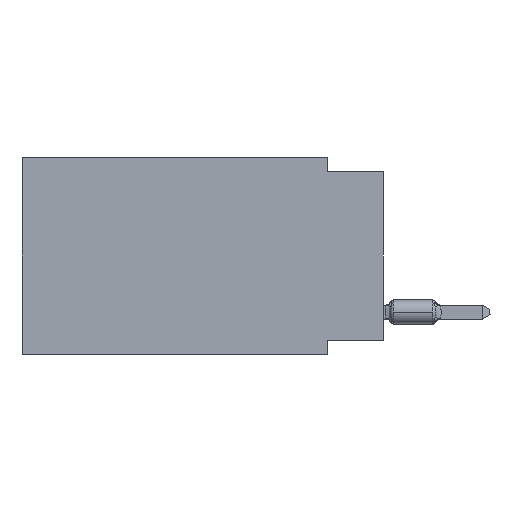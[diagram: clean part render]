
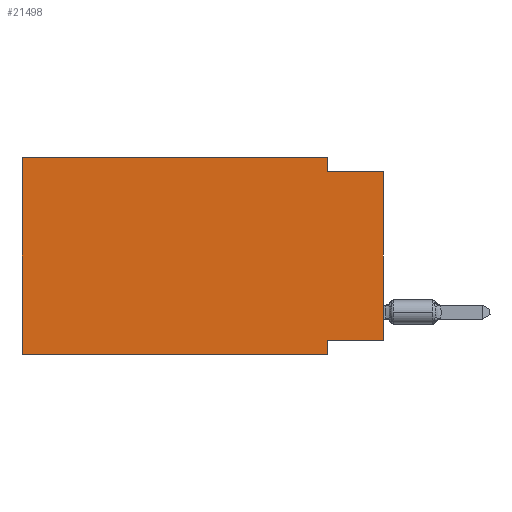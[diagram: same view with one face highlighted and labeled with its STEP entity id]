
A CAD part, left-side view. The second image highlights one B-rep face of the part: STEP entity #21498.
In plain terms, the highlighted planar face has unit normal (-1, 0, 0).
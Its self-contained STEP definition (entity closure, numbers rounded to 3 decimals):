
#720 = CARTESIAN_POINT ( 'NONE',  ( 0., 2.54, -8.255 ) ) ;
#777 = DIRECTION ( 'NONE',  ( 0., 0., 1. ) ) ;
#1091 = EDGE_CURVE ( 'NONE', #18681, #20984, #11143, .T. ) ;
#1257 = DIRECTION ( 'NONE',  ( 0., -1., 0. ) ) ;
#1694 = DIRECTION ( 'NONE',  ( 0., -1., 0. ) ) ;
#2148 = LINE ( 'NONE', #4865, #14960 ) ;
#2224 = CARTESIAN_POINT ( 'NONE',  ( 0., 0., -8.255 ) ) ;
#2436 = EDGE_CURVE ( 'NONE', #14122, #18681, #3145, .T. ) ;
#2626 = CARTESIAN_POINT ( 'NONE',  ( 0., 16.383, -8.89 ) ) ;
#3067 = CARTESIAN_POINT ( 'NONE',  ( 0., 16.383, 0. ) ) ;
#3145 = LINE ( 'NONE', #5214, #20557 ) ;
#3168 = LINE ( 'NONE', #5904, #10382 ) ;
#3316 = ORIENTED_EDGE ( 'NONE', *, *, #2436, .F. ) ;
#3697 = LINE ( 'NONE', #2224, #21418 ) ;
#4865 = CARTESIAN_POINT ( 'NONE',  ( 0., 16.383, -8.89 ) ) ;
#5214 = CARTESIAN_POINT ( 'NONE',  ( 0., 2.54, 0. ) ) ;
#5703 = ORIENTED_EDGE ( 'NONE', *, *, #23258, .F. ) ;
#5904 = CARTESIAN_POINT ( 'NONE',  ( 0., 0., 0. ) ) ;
#6479 = VERTEX_POINT ( 'NONE', #2626 ) ;
#6645 = CARTESIAN_POINT ( 'NONE',  ( 0., 2.54, -8.89 ) ) ;
#7131 = DIRECTION ( 'NONE',  ( 0., 0., -1. ) ) ;
#8596 = CARTESIAN_POINT ( 'NONE',  ( 0., 0., -0.635 ) ) ;
#9257 = CARTESIAN_POINT ( 'NONE',  ( 0., 2.54, 0. ) ) ;
#9400 = DIRECTION ( 'NONE',  ( 0., 1., 0. ) ) ;
#9467 = VECTOR ( 'NONE', #1257, 1000. ) ;
#9841 = VERTEX_POINT ( 'NONE', #3067 ) ;
#10206 = EDGE_CURVE ( 'NONE', #24251, #11737, #21791, .T. ) ;
#10382 = VECTOR ( 'NONE', #25155, 1000. ) ;
#10495 = DIRECTION ( 'NONE',  ( 0., 0., -1. ) ) ;
#10519 = EDGE_CURVE ( 'NONE', #6479, #11737, #2148, .T. ) ;
#11143 = LINE ( 'NONE', #8596, #9467 ) ;
#11737 = VERTEX_POINT ( 'NONE', #6645 ) ;
#12640 = AXIS2_PLACEMENT_3D ( 'NONE', #20639, #26007, #28410 ) ;
#12718 = LINE ( 'NONE', #12869, #29588 ) ;
#12869 = CARTESIAN_POINT ( 'NONE',  ( 0., 16.383, 0. ) ) ;
#13039 = DIRECTION ( 'NONE',  ( 0., -1., 0. ) ) ;
#13054 = ORIENTED_EDGE ( 'NONE', *, *, #26590, .F. ) ;
#13904 = PLANE ( 'NONE',  #12640 ) ;
#13909 = CARTESIAN_POINT ( 'NONE',  ( 0., 2.54, -0.635 ) ) ;
#14122 = VERTEX_POINT ( 'NONE', #9257 ) ;
#14354 = CARTESIAN_POINT ( 'NONE',  ( 0., 0., -8.255 ) ) ;
#14960 = VECTOR ( 'NONE', #1694, 1000. ) ;
#15456 = EDGE_CURVE ( 'NONE', #15779, #20984, #3168, .T. ) ;
#15521 = FACE_OUTER_BOUND ( 'NONE', #19790, .T. ) ;
#15779 = VERTEX_POINT ( 'NONE', #14354 ) ;
#17828 = ORIENTED_EDGE ( 'NONE', *, *, #21966, .F. ) ;
#18048 = ORIENTED_EDGE ( 'NONE', *, *, #10206, .F. ) ;
#18681 = VERTEX_POINT ( 'NONE', #13909 ) ;
#19395 = CARTESIAN_POINT ( 'NONE',  ( 0., 2.54, -8.89 ) ) ;
#19790 = EDGE_LOOP ( 'NONE', ( #25662, #21817, #3316, #13054, #5703, #28491, #18048, #17828 ) ) ;
#20557 = VECTOR ( 'NONE', #10495, 1000. ) ;
#20639 = CARTESIAN_POINT ( 'NONE',  ( 0., 16.383, 0. ) ) ;
#20984 = VERTEX_POINT ( 'NONE', #27330 ) ;
#21115 = VECTOR ( 'NONE', #13039, 1000. ) ;
#21418 = VECTOR ( 'NONE', #9400, 1000. ) ;
#21498 = ADVANCED_FACE ( 'NONE', ( #15521 ), #13904, .F. ) ;
#21791 = LINE ( 'NONE', #19395, #24614 ) ;
#21817 = ORIENTED_EDGE ( 'NONE', *, *, #1091, .F. ) ;
#21966 = EDGE_CURVE ( 'NONE', #15779, #24251, #3697, .T. ) ;
#23258 = EDGE_CURVE ( 'NONE', #6479, #9841, #12718, .T. ) ;
#24251 = VERTEX_POINT ( 'NONE', #720 ) ;
#24614 = VECTOR ( 'NONE', #7131, 1000. ) ;
#24968 = CARTESIAN_POINT ( 'NONE',  ( 0., 16.383, 0. ) ) ;
#25155 = DIRECTION ( 'NONE',  ( 0., 0., 1. ) ) ;
#25662 = ORIENTED_EDGE ( 'NONE', *, *, #15456, .T. ) ;
#26007 = DIRECTION ( 'NONE',  ( 1., 0., 0. ) ) ;
#26590 = EDGE_CURVE ( 'NONE', #9841, #14122, #29752, .T. ) ;
#27330 = CARTESIAN_POINT ( 'NONE',  ( 0., 0., -0.635 ) ) ;
#28410 = DIRECTION ( 'NONE',  ( 0., 0., -1. ) ) ;
#28491 = ORIENTED_EDGE ( 'NONE', *, *, #10519, .T. ) ;
#29588 = VECTOR ( 'NONE', #777, 1000. ) ;
#29752 = LINE ( 'NONE', #24968, #21115 ) ;
